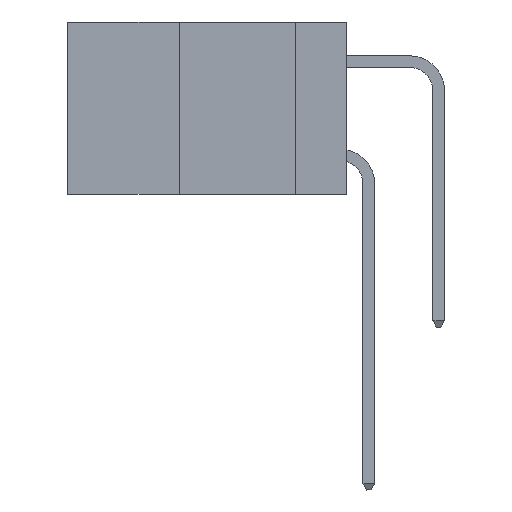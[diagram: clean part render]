
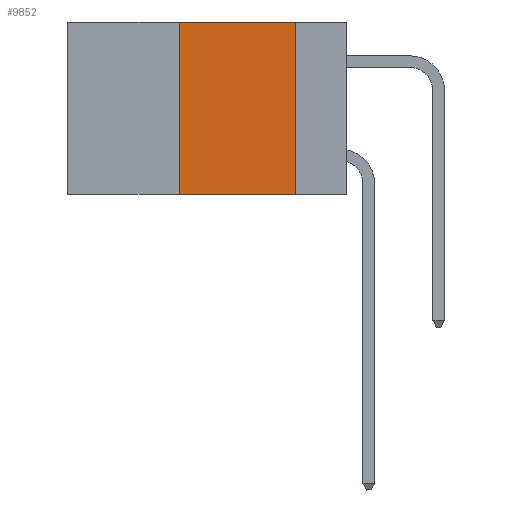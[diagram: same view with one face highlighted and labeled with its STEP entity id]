
A CAD part, left-side view. The second image highlights one B-rep face of the part: STEP entity #9852.
In plain terms, the highlighted planar face has unit normal (-1, 0, 0).
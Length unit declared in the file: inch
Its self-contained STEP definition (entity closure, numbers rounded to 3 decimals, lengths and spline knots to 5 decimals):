
#367 = FACE_OUTER_BOUND ( 'NONE', #2617, .T. ) ;
#764 = DIRECTION ( 'NONE',  ( 0., -1., 0. ) ) ;
#1788 = CARTESIAN_POINT ( 'NONE',  ( 0., 0.11, 0. ) ) ;
#2617 = EDGE_LOOP ( 'NONE', ( #9625, #10777, #8217, #14030 ) ) ;
#3087 = DIRECTION ( 'NONE',  ( 0., 0., -1. ) ) ;
#3449 = LINE ( 'NONE', #5852, #10188 ) ;
#3476 = VERTEX_POINT ( 'NONE', #10070 ) ;
#3574 = CARTESIAN_POINT ( 'NONE',  ( 0., 0.36, -0.37 ) ) ;
#3644 = DIRECTION ( 'NONE',  ( 0., 0., 1. ) ) ;
#4468 = CARTESIAN_POINT ( 'NONE',  ( 0., 0.11, -0.37 ) ) ;
#5262 = VECTOR ( 'NONE', #764, 39.37008 ) ;
#5294 = DIRECTION ( 'NONE',  ( 1., 0., 0. ) ) ;
#5481 = CARTESIAN_POINT ( 'NONE',  ( 0., 0.6, -0.37 ) ) ;
#5852 = CARTESIAN_POINT ( 'NONE',  ( 0., 0.36, 0. ) ) ;
#6423 = DIRECTION ( 'NONE',  ( 0., 0., -1. ) ) ;
#6434 = EDGE_CURVE ( 'NONE', #7667, #11580, #12002, .T. ) ;
#7261 = EDGE_CURVE ( 'NONE', #13556, #3476, #3449, .T. ) ;
#7667 = VERTEX_POINT ( 'NONE', #1788 ) ;
#8217 = ORIENTED_EDGE ( 'NONE', *, *, #7261, .F. ) ;
#8299 = AXIS2_PLACEMENT_3D ( 'NONE', #8765, #5294, #6423 ) ;
#8419 = DIRECTION ( 'NONE',  ( 0., -1., 0. ) ) ;
#8765 = CARTESIAN_POINT ( 'NONE',  ( 0., 0.6, 0. ) ) ;
#9400 = EDGE_CURVE ( 'NONE', #13556, #11580, #14219, .T. ) ;
#9625 = ORIENTED_EDGE ( 'NONE', *, *, #6434, .F. ) ;
#9852 = ADVANCED_FACE ( 'NONE', ( #367 ), #11746, .F. ) ;
#10070 = CARTESIAN_POINT ( 'NONE',  ( 0., 0.36, 0. ) ) ;
#10089 = LINE ( 'NONE', #11676, #10805 ) ;
#10188 = VECTOR ( 'NONE', #3644, 39.37008 ) ;
#10777 = ORIENTED_EDGE ( 'NONE', *, *, #13846, .F. ) ;
#10805 = VECTOR ( 'NONE', #8419, 39.37008 ) ;
#11580 = VERTEX_POINT ( 'NONE', #4468 ) ;
#11630 = VECTOR ( 'NONE', #3087, 39.37008 ) ;
#11676 = CARTESIAN_POINT ( 'NONE',  ( 0., 0.6, 0. ) ) ;
#11746 = PLANE ( 'NONE',  #8299 ) ;
#12002 = LINE ( 'NONE', #13231, #11630 ) ;
#13231 = CARTESIAN_POINT ( 'NONE',  ( 0., 0.11, 0. ) ) ;
#13556 = VERTEX_POINT ( 'NONE', #3574 ) ;
#13846 = EDGE_CURVE ( 'NONE', #3476, #7667, #10089, .T. ) ;
#14030 = ORIENTED_EDGE ( 'NONE', *, *, #9400, .T. ) ;
#14219 = LINE ( 'NONE', #5481, #5262 ) ;
